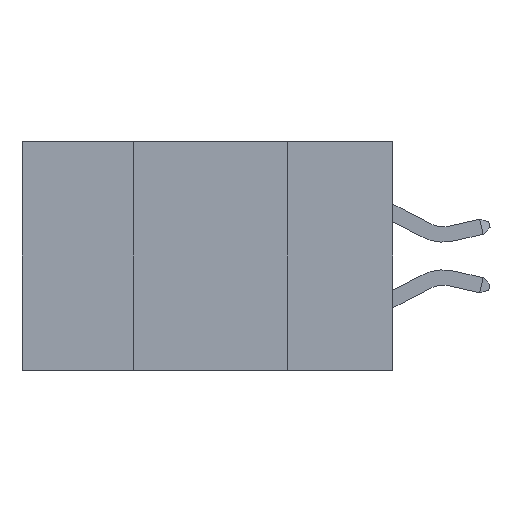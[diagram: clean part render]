
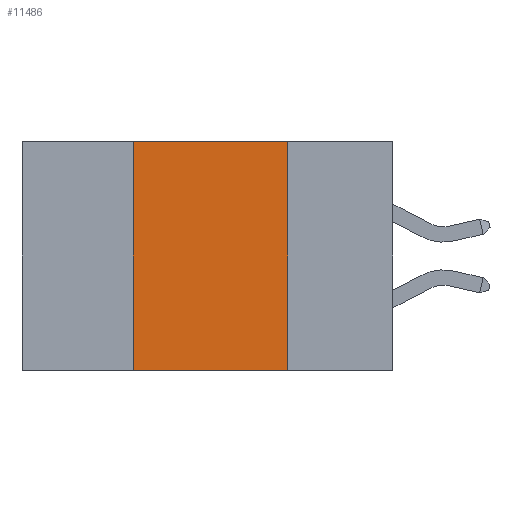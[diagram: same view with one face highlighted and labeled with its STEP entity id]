
A CAD part, left-side view. The second image highlights one B-rep face of the part: STEP entity #11486.
In plain terms, the highlighted planar face has unit normal (-1, 0, 0).
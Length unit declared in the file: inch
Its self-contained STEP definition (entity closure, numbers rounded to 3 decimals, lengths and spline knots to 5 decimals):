
#639 = VECTOR ( 'NONE', #4384, 39.37008 ) ;
#670 = VERTEX_POINT ( 'NONE', #1867 ) ;
#790 = FACE_OUTER_BOUND ( 'NONE', #8209, .T. ) ;
#1085 = AXIS2_PLACEMENT_3D ( 'NONE', #7175, #13251, #11317 ) ;
#1245 = LINE ( 'NONE', #3171, #12553 ) ;
#1328 = CARTESIAN_POINT ( 'NONE',  ( 0., 0.6, 0. ) ) ;
#1803 = ORIENTED_EDGE ( 'NONE', *, *, #6207, .F. ) ;
#1867 = CARTESIAN_POINT ( 'NONE',  ( 0., 0.17, -0.37 ) ) ;
#3171 = CARTESIAN_POINT ( 'NONE',  ( 0., 0.17, 0. ) ) ;
#3243 = LINE ( 'NONE', #1328, #7483 ) ;
#3263 = CARTESIAN_POINT ( 'NONE',  ( 0., 0.42, -0.37 ) ) ;
#3864 = CARTESIAN_POINT ( 'NONE',  ( 0., 0.42, 0. ) ) ;
#3914 = DIRECTION ( 'NONE',  ( 0., 0., 1. ) ) ;
#3998 = ORIENTED_EDGE ( 'NONE', *, *, #10597, .F. ) ;
#4384 = DIRECTION ( 'NONE',  ( 0., -1., 0. ) ) ;
#4876 = EDGE_CURVE ( 'NONE', #11599, #670, #12507, .T. ) ;
#4979 = PLANE ( 'NONE',  #1085 ) ;
#5016 = LINE ( 'NONE', #6251, #10273 ) ;
#6207 = EDGE_CURVE ( 'NONE', #9970, #670, #1245, .T. ) ;
#6251 = CARTESIAN_POINT ( 'NONE',  ( 0., 0.42, 0. ) ) ;
#6845 = ORIENTED_EDGE ( 'NONE', *, *, #4876, .T. ) ;
#6886 = ORIENTED_EDGE ( 'NONE', *, *, #8976, .F. ) ;
#7175 = CARTESIAN_POINT ( 'NONE',  ( 0., 0.6, 0. ) ) ;
#7274 = CARTESIAN_POINT ( 'NONE',  ( 0., 0.6, -0.37 ) ) ;
#7364 = DIRECTION ( 'NONE',  ( 0., -1., 0. ) ) ;
#7483 = VECTOR ( 'NONE', #7364, 39.37008 ) ;
#8209 = EDGE_LOOP ( 'NONE', ( #1803, #6886, #3998, #6845 ) ) ;
#8976 = EDGE_CURVE ( 'NONE', #11882, #9970, #3243, .T. ) ;
#9348 = DIRECTION ( 'NONE',  ( 0., 0., -1. ) ) ;
#9970 = VERTEX_POINT ( 'NONE', #10898 ) ;
#10273 = VECTOR ( 'NONE', #3914, 39.37008 ) ;
#10597 = EDGE_CURVE ( 'NONE', #11599, #11882, #5016, .T. ) ;
#10898 = CARTESIAN_POINT ( 'NONE',  ( 0., 0.17, 0. ) ) ;
#11317 = DIRECTION ( 'NONE',  ( 0., 0., -1. ) ) ;
#11486 = ADVANCED_FACE ( 'NONE', ( #790 ), #4979, .F. ) ;
#11599 = VERTEX_POINT ( 'NONE', #3263 ) ;
#11882 = VERTEX_POINT ( 'NONE', #3864 ) ;
#12507 = LINE ( 'NONE', #7274, #639 ) ;
#12553 = VECTOR ( 'NONE', #9348, 39.37008 ) ;
#13251 = DIRECTION ( 'NONE',  ( 1., 0., 0. ) ) ;
